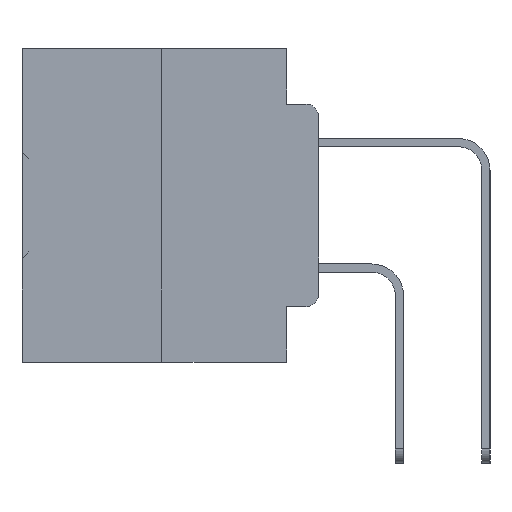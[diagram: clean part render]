
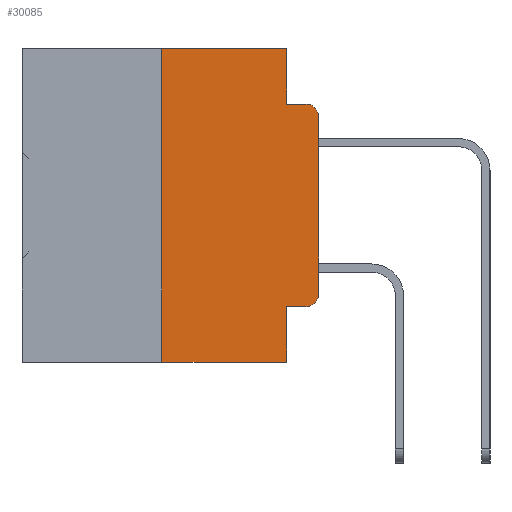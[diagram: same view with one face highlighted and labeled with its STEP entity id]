
A CAD part, left-side view. The second image highlights one B-rep face of the part: STEP entity #30085.
In plain terms, the highlighted planar face has unit normal (-1, 0, 0).
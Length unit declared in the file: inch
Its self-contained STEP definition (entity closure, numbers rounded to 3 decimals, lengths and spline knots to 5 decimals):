
#459 = VERTEX_POINT ( 'NONE', #23507 ) ;
#1340 = VECTOR ( 'NONE', #24269, 39.37008 ) ;
#1545 = LINE ( 'NONE', #3409, #39612 ) ;
#2562 = VECTOR ( 'NONE', #4236, 39.37008 ) ;
#2563 = VERTEX_POINT ( 'NONE', #7216 ) ;
#3409 = CARTESIAN_POINT ( 'NONE',  ( 0., 0.25, 0. ) ) ;
#3547 = LINE ( 'NONE', #34985, #2562 ) ;
#3648 = DIRECTION ( 'NONE',  ( 0., 0., -1. ) ) ;
#4236 = DIRECTION ( 'NONE',  ( 0., -1., 0. ) ) ;
#4966 = EDGE_CURVE ( 'NONE', #18664, #21860, #9200, .T. ) ;
#5618 = EDGE_CURVE ( 'NONE', #2563, #25570, #9638, .T. ) ;
#5721 = VERTEX_POINT ( 'NONE', #24660 ) ;
#7216 = CARTESIAN_POINT ( 'NONE',  ( 0., 0.051, -0.4115 ) ) ;
#7468 = VERTEX_POINT ( 'NONE', #18219 ) ;
#7617 = ORIENTED_EDGE ( 'NONE', *, *, #14019, .F. ) ;
#8226 = EDGE_CURVE ( 'NONE', #26345, #10606, #21583, .T. ) ;
#8517 = EDGE_CURVE ( 'NONE', #459, #7468, #3547, .T. ) ;
#9032 = CARTESIAN_POINT ( 'NONE',  ( 0., 0.051, 0. ) ) ;
#9068 = VECTOR ( 'NONE', #3648, 39.37008 ) ;
#9200 = LINE ( 'NONE', #18538, #24731 ) ;
#9638 = LINE ( 'NONE', #30685, #1340 ) ;
#10239 = DIRECTION ( 'NONE',  ( -1., 0., 0. ) ) ;
#10422 = CIRCLE ( 'NONE', #11375, 0.02 ) ;
#10568 = ORIENTED_EDGE ( 'NONE', *, *, #5618, .T. ) ;
#10606 = VERTEX_POINT ( 'NONE', #16377 ) ;
#11375 = AXIS2_PLACEMENT_3D ( 'NONE', #28744, #10239, #31807 ) ;
#11833 = DIRECTION ( 'NONE',  ( 1., 0., 0. ) ) ;
#12202 = DIRECTION ( 'NONE',  ( 0., 0., -1. ) ) ;
#12368 = VECTOR ( 'NONE', #27812, 39.37008 ) ;
#12417 = EDGE_LOOP ( 'NONE', ( #21227, #25996, #36976, #21744, #39831, #13039, #31315, #7617, #10568, #14920 ) ) ;
#13039 = ORIENTED_EDGE ( 'NONE', *, *, #22334, .F. ) ;
#13088 = CARTESIAN_POINT ( 'NONE',  ( 0., 0.051, 0. ) ) ;
#13824 = CARTESIAN_POINT ( 'NONE',  ( 0., 0.051, -0.0885 ) ) ;
#14019 = EDGE_CURVE ( 'NONE', #2563, #7468, #15297, .T. ) ;
#14837 = CARTESIAN_POINT ( 'NONE',  ( 0., 0.473, 0. ) ) ;
#14920 = ORIENTED_EDGE ( 'NONE', *, *, #37344, .T. ) ;
#15106 = VECTOR ( 'NONE', #16934, 39.37008 ) ;
#15297 = LINE ( 'NONE', #9032, #38754 ) ;
#15953 = DIRECTION ( 'NONE',  ( 0., 0., 1. ) ) ;
#16377 = CARTESIAN_POINT ( 'NONE',  ( 0., 0., -0.1085 ) ) ;
#16820 = CARTESIAN_POINT ( 'NONE',  ( 0., 0.02, -0.3915 ) ) ;
#16934 = DIRECTION ( 'NONE',  ( 0., -1., 0. ) ) ;
#18219 = CARTESIAN_POINT ( 'NONE',  ( 0., 0.051, -0.5 ) ) ;
#18538 = CARTESIAN_POINT ( 'NONE',  ( 0., 0.473, 0. ) ) ;
#18664 = VERTEX_POINT ( 'NONE', #25327 ) ;
#19456 = EDGE_CURVE ( 'NONE', #23048, #5721, #39512, .T. ) ;
#19919 = DIRECTION ( 'NONE',  ( 0., 0., -1. ) ) ;
#21227 = ORIENTED_EDGE ( 'NONE', *, *, #8226, .T. ) ;
#21583 = LINE ( 'NONE', #24754, #12368 ) ;
#21744 = ORIENTED_EDGE ( 'NONE', *, *, #36596, .F. ) ;
#21860 = VERTEX_POINT ( 'NONE', #37508 ) ;
#22334 = EDGE_CURVE ( 'NONE', #459, #18664, #1545, .T. ) ;
#23048 = VERTEX_POINT ( 'NONE', #37558 ) ;
#23488 = AXIS2_PLACEMENT_3D ( 'NONE', #14837, #11833, #33345 ) ;
#23507 = CARTESIAN_POINT ( 'NONE',  ( 0., 0.25, -0.5 ) ) ;
#24139 = PLANE ( 'NONE',  #23488 ) ;
#24269 = DIRECTION ( 'NONE',  ( 0., -1., 0. ) ) ;
#24660 = CARTESIAN_POINT ( 'NONE',  ( 0., 0.02, -0.0885 ) ) ;
#24725 = DIRECTION ( 'NONE',  ( 0., -1., 0. ) ) ;
#24731 = VECTOR ( 'NONE', #24725, 39.37008 ) ;
#24754 = CARTESIAN_POINT ( 'NONE',  ( 0., 0., 0. ) ) ;
#25327 = CARTESIAN_POINT ( 'NONE',  ( 0., 0.25, 0. ) ) ;
#25541 = LINE ( 'NONE', #13088, #9068 ) ;
#25570 = VERTEX_POINT ( 'NONE', #27838 ) ;
#25996 = ORIENTED_EDGE ( 'NONE', *, *, #33795, .T. ) ;
#26345 = VERTEX_POINT ( 'NONE', #28051 ) ;
#26695 = AXIS2_PLACEMENT_3D ( 'NONE', #16820, #38185, #19919 ) ;
#27812 = DIRECTION ( 'NONE',  ( 0., 0., 1. ) ) ;
#27838 = CARTESIAN_POINT ( 'NONE',  ( 0., 0.02, -0.4115 ) ) ;
#28051 = CARTESIAN_POINT ( 'NONE',  ( 0., 0., -0.3915 ) ) ;
#28135 = FACE_OUTER_BOUND ( 'NONE', #12417, .T. ) ;
#28744 = CARTESIAN_POINT ( 'NONE',  ( 0., 0.02, -0.1085 ) ) ;
#30085 = ADVANCED_FACE ( 'NONE', ( #28135 ), #24139, .F. ) ;
#30685 = CARTESIAN_POINT ( 'NONE',  ( 0., 0.051, -0.4115 ) ) ;
#31315 = ORIENTED_EDGE ( 'NONE', *, *, #8517, .T. ) ;
#31807 = DIRECTION ( 'NONE',  ( 0., 0., -1. ) ) ;
#33345 = DIRECTION ( 'NONE',  ( 0., 0., -1. ) ) ;
#33795 = EDGE_CURVE ( 'NONE', #10606, #5721, #10422, .T. ) ;
#34985 = CARTESIAN_POINT ( 'NONE',  ( 0., 0.473, -0.5 ) ) ;
#36445 = CIRCLE ( 'NONE', #26695, 0.02 ) ;
#36596 = EDGE_CURVE ( 'NONE', #21860, #23048, #25541, .T. ) ;
#36976 = ORIENTED_EDGE ( 'NONE', *, *, #19456, .F. ) ;
#37344 = EDGE_CURVE ( 'NONE', #25570, #26345, #36445, .T. ) ;
#37508 = CARTESIAN_POINT ( 'NONE',  ( 0., 0.051, 0. ) ) ;
#37558 = CARTESIAN_POINT ( 'NONE',  ( 0., 0.051, -0.0885 ) ) ;
#38185 = DIRECTION ( 'NONE',  ( -1., 0., 0. ) ) ;
#38754 = VECTOR ( 'NONE', #12202, 39.37008 ) ;
#39512 = LINE ( 'NONE', #13824, #15106 ) ;
#39612 = VECTOR ( 'NONE', #15953, 39.37008 ) ;
#39831 = ORIENTED_EDGE ( 'NONE', *, *, #4966, .F. ) ;
